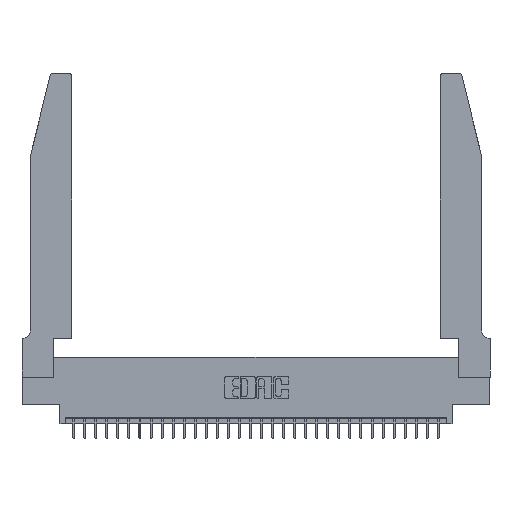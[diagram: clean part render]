
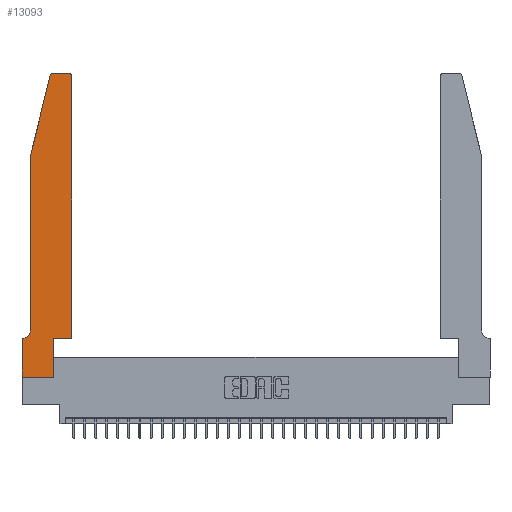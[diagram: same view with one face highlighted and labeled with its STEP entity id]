
A CAD part, top view. The second image highlights one B-rep face of the part: STEP entity #13093.
In plain terms, the highlighted planar face has unit normal (0, 0, 1).
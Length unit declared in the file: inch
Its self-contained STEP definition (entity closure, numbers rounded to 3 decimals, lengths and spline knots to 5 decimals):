
#127 = VERTEX_POINT ( 'NONE', #736 ) ;
#247 = DIRECTION ( 'NONE',  ( 0., 0., 1. ) ) ;
#736 = CARTESIAN_POINT ( 'NONE',  ( 0., 0., 0.37 ) ) ;
#762 = ORIENTED_EDGE ( 'NONE', *, *, #29529, .T. ) ;
#1130 = ORIENTED_EDGE ( 'NONE', *, *, #30111, .T. ) ;
#1642 = DIRECTION ( 'NONE',  ( 0., 1., 0. ) ) ;
#3051 = CARTESIAN_POINT ( 'NONE',  ( 0.0055, 0.35, 0.37 ) ) ;
#3171 = VECTOR ( 'NONE', #26675, 39.37008 ) ;
#3346 = EDGE_CURVE ( 'NONE', #28154, #28665, #17392, .T. ) ;
#3570 = VECTOR ( 'NONE', #22760, 39.37008 ) ;
#3612 = CARTESIAN_POINT ( 'NONE',  ( 0.0755, 0.35, 0.37 ) ) ;
#3823 = ORIENTED_EDGE ( 'NONE', *, *, #16799, .T. ) ;
#3835 = EDGE_LOOP ( 'NONE', ( #1130, #3823, #7553, #28641, #19815, #6002, #12924, #26558, #12660, #6758, #762, #6609 ) ) ;
#3952 = CARTESIAN_POINT ( 'NONE',  ( 0., 0.35, 0.37 ) ) ;
#4131 = CARTESIAN_POINT ( 'NONE',  ( 0.4205, 2.72, 0.37 ) ) ;
#5375 = CARTESIAN_POINT ( 'NONE',  ( 0.2605, 2.75, 0.37 ) ) ;
#6002 = ORIENTED_EDGE ( 'NONE', *, *, #31141, .T. ) ;
#6609 = ORIENTED_EDGE ( 'NONE', *, *, #23764, .T. ) ;
#6697 = VECTOR ( 'NONE', #23870, 39.37008 ) ;
#6758 = ORIENTED_EDGE ( 'NONE', *, *, #14309, .T. ) ;
#6992 = CARTESIAN_POINT ( 'NONE',  ( 0.0755, 0.42, 0.37 ) ) ;
#7146 = DIRECTION ( 'NONE',  ( -0.239, -0.971, 0. ) ) ;
#7387 = VERTEX_POINT ( 'NONE', #10751 ) ;
#7455 = VERTEX_POINT ( 'NONE', #23502 ) ;
#7462 = DIRECTION ( 'NONE',  ( 0., 0., -1. ) ) ;
#7538 = EDGE_CURVE ( 'NONE', #28665, #13867, #8610, .T. ) ;
#7553 = ORIENTED_EDGE ( 'NONE', *, *, #3346, .T. ) ;
#8178 = LINE ( 'NONE', #5375, #3570 ) ;
#8184 = VECTOR ( 'NONE', #1642, 39.37008 ) ;
#8610 = LINE ( 'NONE', #21191, #24701 ) ;
#9075 = LINE ( 'NONE', #14204, #8184 ) ;
#9370 = DIRECTION ( 'NONE',  ( 0., -1., 0. ) ) ;
#9918 = DIRECTION ( 'NONE',  ( -1., 0., 0. ) ) ;
#10751 = CARTESIAN_POINT ( 'NONE',  ( 0.284, 2.75, 0.37 ) ) ;
#11437 = CARTESIAN_POINT ( 'NONE',  ( 0.2865, 0.35, 0.37 ) ) ;
#11450 = LINE ( 'NONE', #18570, #3171 ) ;
#11755 = DIRECTION ( 'NONE',  ( 0., 0., 1. ) ) ;
#11944 = CARTESIAN_POINT ( 'NONE',  ( 0.0755, 2., 0.37 ) ) ;
#11996 = CARTESIAN_POINT ( 'NONE',  ( 0.4205, 2.75, 0.37 ) ) ;
#12627 = VECTOR ( 'NONE', #23488, 39.37008 ) ;
#12660 = ORIENTED_EDGE ( 'NONE', *, *, #16833, .T. ) ;
#12824 = DIRECTION ( 'NONE',  ( 1., 0., 0. ) ) ;
#12924 = ORIENTED_EDGE ( 'NONE', *, *, #13617, .T. ) ;
#13093 = ADVANCED_FACE ( 'NONE', ( #18436 ), #30552, .T. ) ;
#13617 = EDGE_CURVE ( 'NONE', #29467, #127, #11450, .T. ) ;
#13860 = VERTEX_POINT ( 'NONE', #19562 ) ;
#13867 = VERTEX_POINT ( 'NONE', #6992 ) ;
#14204 = CARTESIAN_POINT ( 'NONE',  ( 0.4505, 0.35, 0.37 ) ) ;
#14301 = AXIS2_PLACEMENT_3D ( 'NONE', #4131, #11755, #21858 ) ;
#14309 = EDGE_CURVE ( 'NONE', #28012, #7455, #29919, .T. ) ;
#14634 = VERTEX_POINT ( 'NONE', #20166 ) ;
#16240 = LINE ( 'NONE', #11437, #6697 ) ;
#16799 = EDGE_CURVE ( 'NONE', #7387, #28154, #18281, .T. ) ;
#16833 = EDGE_CURVE ( 'NONE', #14634, #28012, #16240, .T. ) ;
#17392 = LINE ( 'NONE', #11944, #23993 ) ;
#17712 = CARTESIAN_POINT ( 'NONE',  ( 0.0055, 0.42, 0.37 ) ) ;
#17759 = LINE ( 'NONE', #19759, #29616 ) ;
#18281 = CIRCLE ( 'NONE', #32620, 0.03 ) ;
#18436 = FACE_OUTER_BOUND ( 'NONE', #3835, .T. ) ;
#18439 = DIRECTION ( 'NONE',  ( 1., 0., 0. ) ) ;
#18570 = CARTESIAN_POINT ( 'NONE',  ( 0., 0., 0.37 ) ) ;
#19562 = CARTESIAN_POINT ( 'NONE',  ( 0.4505, 2.72, 0.37 ) ) ;
#19759 = CARTESIAN_POINT ( 'NONE',  ( 0., 0., 0.37 ) ) ;
#19815 = ORIENTED_EDGE ( 'NONE', *, *, #29151, .T. ) ;
#20166 = CARTESIAN_POINT ( 'NONE',  ( 0.2865, 0., 0.37 ) ) ;
#21191 = CARTESIAN_POINT ( 'NONE',  ( 0.0755, 2., 0.37 ) ) ;
#21675 = AXIS2_PLACEMENT_3D ( 'NONE', #30889, #247, #12824 ) ;
#21858 = DIRECTION ( 'NONE',  ( 1., 0., 0. ) ) ;
#22374 = CIRCLE ( 'NONE', #26581, 0.07 ) ;
#22760 = DIRECTION ( 'NONE',  ( -1., 0., 0. ) ) ;
#22856 = VERTEX_POINT ( 'NONE', #11996 ) ;
#23000 = EDGE_CURVE ( 'NONE', #127, #14634, #17759, .T. ) ;
#23488 = DIRECTION ( 'NONE',  ( -1., 0., 0. ) ) ;
#23502 = CARTESIAN_POINT ( 'NONE',  ( 0.4505, 0.35, 0.37 ) ) ;
#23764 = EDGE_CURVE ( 'NONE', #13860, #22856, #31254, .T. ) ;
#23870 = DIRECTION ( 'NONE',  ( 0., 1., 0. ) ) ;
#23946 = CARTESIAN_POINT ( 'NONE',  ( 0.0755, 2., 0.37 ) ) ;
#23993 = VECTOR ( 'NONE', #7146, 39.37008 ) ;
#24338 = VERTEX_POINT ( 'NONE', #3051 ) ;
#24701 = VECTOR ( 'NONE', #9370, 39.37008 ) ;
#25501 = CARTESIAN_POINT ( 'NONE',  ( 0.284, 2.72, 0.37 ) ) ;
#26284 = LINE ( 'NONE', #3612, #12627 ) ;
#26558 = ORIENTED_EDGE ( 'NONE', *, *, #23000, .T. ) ;
#26581 = AXIS2_PLACEMENT_3D ( 'NONE', #17712, #7462, #9918 ) ;
#26675 = DIRECTION ( 'NONE',  ( 0., -1., 0. ) ) ;
#27408 = CARTESIAN_POINT ( 'NONE',  ( 0.4505, 0.35, 0.37 ) ) ;
#28012 = VERTEX_POINT ( 'NONE', #29977 ) ;
#28151 = DIRECTION ( 'NONE',  ( 1., 0., 0. ) ) ;
#28154 = VERTEX_POINT ( 'NONE', #28433 ) ;
#28433 = CARTESIAN_POINT ( 'NONE',  ( 0.25487, 2.72718, 0.37 ) ) ;
#28641 = ORIENTED_EDGE ( 'NONE', *, *, #7538, .T. ) ;
#28665 = VERTEX_POINT ( 'NONE', #23946 ) ;
#29151 = EDGE_CURVE ( 'NONE', #13867, #24338, #22374, .T. ) ;
#29467 = VERTEX_POINT ( 'NONE', #3952 ) ;
#29529 = EDGE_CURVE ( 'NONE', #7455, #13860, #9075, .T. ) ;
#29616 = VECTOR ( 'NONE', #29882, 39.37008 ) ;
#29882 = DIRECTION ( 'NONE',  ( 1., 0., 0. ) ) ;
#29919 = LINE ( 'NONE', #27408, #31264 ) ;
#29977 = CARTESIAN_POINT ( 'NONE',  ( 0.2865, 0.35, 0.37 ) ) ;
#30111 = EDGE_CURVE ( 'NONE', #22856, #7387, #8178, .T. ) ;
#30552 = PLANE ( 'NONE',  #21675 ) ;
#30889 = CARTESIAN_POINT ( 'NONE',  ( 0., 0.35, 0.37 ) ) ;
#31141 = EDGE_CURVE ( 'NONE', #24338, #29467, #26284, .T. ) ;
#31254 = CIRCLE ( 'NONE', #14301, 0.03 ) ;
#31264 = VECTOR ( 'NONE', #18439, 39.37008 ) ;
#32567 = DIRECTION ( 'NONE',  ( 0., 0., 1. ) ) ;
#32620 = AXIS2_PLACEMENT_3D ( 'NONE', #25501, #32567, #28151 ) ;
